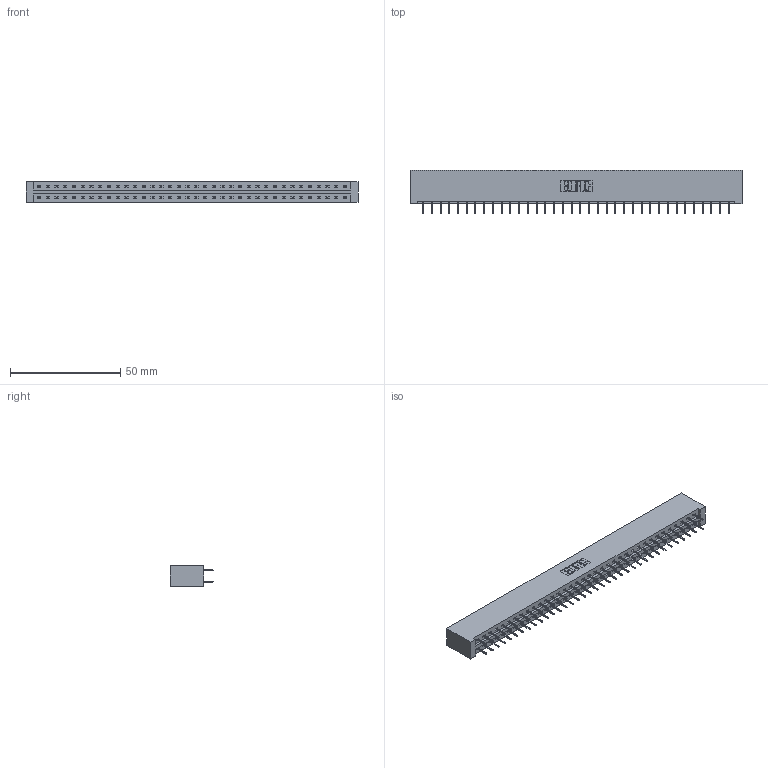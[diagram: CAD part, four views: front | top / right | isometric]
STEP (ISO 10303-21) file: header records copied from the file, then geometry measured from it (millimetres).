
FILE_DESCRIPTION (( 'STEP AP203' ), '1' );
FILE_NAME ('387-072-524-201.STEP', '2018-09-22T18:01:17', ( '' ), ( '' ), 'SwSTEP 2.0', 'SolidWorks 2016', '' );
FILE_SCHEMA (( 'CONFIG_CONTROL_DESIGN' ));
Length unit declared in the file: inch
Products named in the file (3): 337 Part_No Mounting Lugs; 345-292-001_345-293-124; 387-072-524-201
Assembly tree (73 placements, depth 2):
  387-072-524-201
    337 Part_No Mounting Lugs
    345-292-001_345-293-124  x72
Bounding box: 150.52 x 19.69 x 9.4 mm (x, y, z)
Volume: 16434.9 mm3; surface area: 18240.1 mm2
Topology: 73 solids, 73 shells, 4282 faces, 12167 edges, 7822 vertices
Faces by surface type: plane 3234, cylinder 1048
Entity records: 28485 total; most frequent: CARTESIAN_POINT 4802, ORIENTED_EDGE 4738, DIRECTION 4089, EDGE_CURVE 2369, LINE 2253, VECTOR 2253, VERTEX_POINT 1574, AXIS2_PLACEMENT_3D 918
